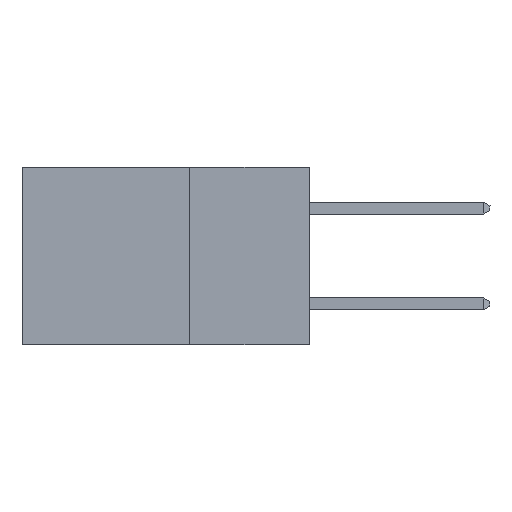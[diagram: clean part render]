
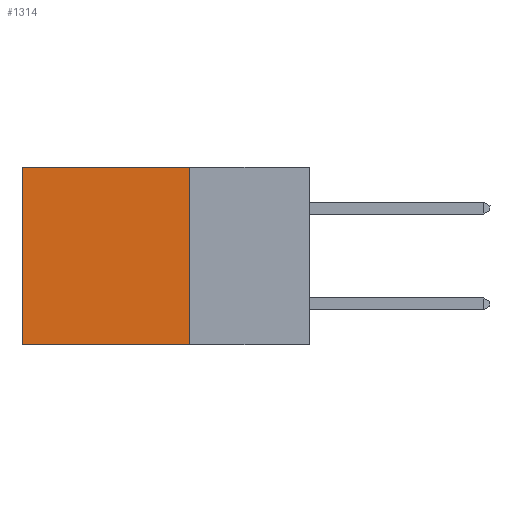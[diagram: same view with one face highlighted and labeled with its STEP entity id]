
A CAD part, left-side view. The second image highlights one B-rep face of the part: STEP entity #1314.
In plain terms, the highlighted planar face has unit normal (-1, 0, 0).
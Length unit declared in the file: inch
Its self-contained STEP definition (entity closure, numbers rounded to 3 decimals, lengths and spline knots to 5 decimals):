
#69 = CARTESIAN_POINT ( 'NONE',  ( 0.2875, 0.25, 0. ) ) ;
#151 = EDGE_CURVE ( 'NONE', #1195, #3680, #4042, .T. ) ;
#1141 = EDGE_CURVE ( 'NONE', #3680, #5228, #1753, .T. ) ;
#1195 = VERTEX_POINT ( 'NONE', #8720 ) ;
#1314 = ADVANCED_FACE ( 'NONE', ( #12053 ), #8704, .F. ) ;
#1459 = LINE ( 'NONE', #10713, #6401 ) ;
#1620 = DIRECTION ( 'NONE',  ( 1., 0., 0. ) ) ;
#1692 = CARTESIAN_POINT ( 'NONE',  ( 0.2875, 0.6, 0. ) ) ;
#1753 = LINE ( 'NONE', #9830, #11403 ) ;
#2761 = CARTESIAN_POINT ( 'NONE',  ( 0.2875, 0.25, 0. ) ) ;
#2836 = AXIS2_PLACEMENT_3D ( 'NONE', #69, #1620, #4730 ) ;
#3680 = VERTEX_POINT ( 'NONE', #1692 ) ;
#3761 = VECTOR ( 'NONE', #11863, 39.37008 ) ;
#4042 = LINE ( 'NONE', #2761, #3761 ) ;
#4313 = EDGE_CURVE ( 'NONE', #4488, #5228, #10797, .T. ) ;
#4488 = VERTEX_POINT ( 'NONE', #4696 ) ;
#4652 = ORIENTED_EDGE ( 'NONE', *, *, #10039, .F. ) ;
#4696 = CARTESIAN_POINT ( 'NONE',  ( 0.2875, 0.25, -0.37 ) ) ;
#4730 = DIRECTION ( 'NONE',  ( 0., 0., -1. ) ) ;
#5228 = VERTEX_POINT ( 'NONE', #12016 ) ;
#6401 = VECTOR ( 'NONE', #6896, 39.37008 ) ;
#6744 = ORIENTED_EDGE ( 'NONE', *, *, #4313, .F. ) ;
#6896 = DIRECTION ( 'NONE',  ( 0., 0., -1. ) ) ;
#6998 = CARTESIAN_POINT ( 'NONE',  ( 0.2875, 0.25, -0.37 ) ) ;
#8175 = DIRECTION ( 'NONE',  ( 0., 1., 0. ) ) ;
#8279 = VECTOR ( 'NONE', #8175, 39.37008 ) ;
#8704 = PLANE ( 'NONE',  #2836 ) ;
#8717 = ORIENTED_EDGE ( 'NONE', *, *, #1141, .T. ) ;
#8720 = CARTESIAN_POINT ( 'NONE',  ( 0.2875, 0.25, 0. ) ) ;
#9380 = EDGE_LOOP ( 'NONE', ( #8717, #6744, #4652, #12006 ) ) ;
#9830 = CARTESIAN_POINT ( 'NONE',  ( 0.2875, 0.6, 0. ) ) ;
#10039 = EDGE_CURVE ( 'NONE', #1195, #4488, #1459, .T. ) ;
#10713 = CARTESIAN_POINT ( 'NONE',  ( 0.2875, 0.25, 0. ) ) ;
#10797 = LINE ( 'NONE', #6998, #8279 ) ;
#11403 = VECTOR ( 'NONE', #12005, 39.37008 ) ;
#11863 = DIRECTION ( 'NONE',  ( 0., 1., 0. ) ) ;
#12005 = DIRECTION ( 'NONE',  ( 0., 0., -1. ) ) ;
#12006 = ORIENTED_EDGE ( 'NONE', *, *, #151, .T. ) ;
#12016 = CARTESIAN_POINT ( 'NONE',  ( 0.2875, 0.6, -0.37 ) ) ;
#12053 = FACE_OUTER_BOUND ( 'NONE', #9380, .T. ) ;
